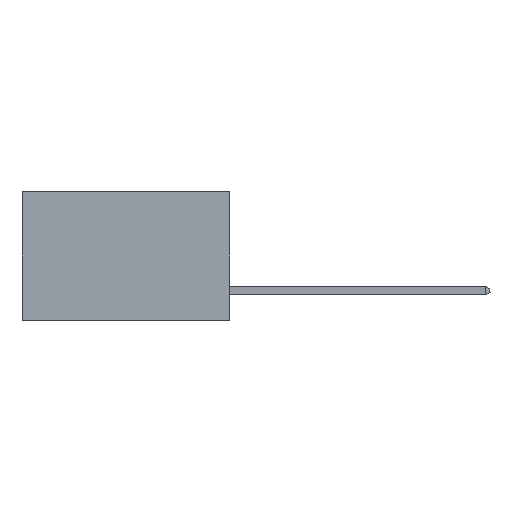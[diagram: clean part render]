
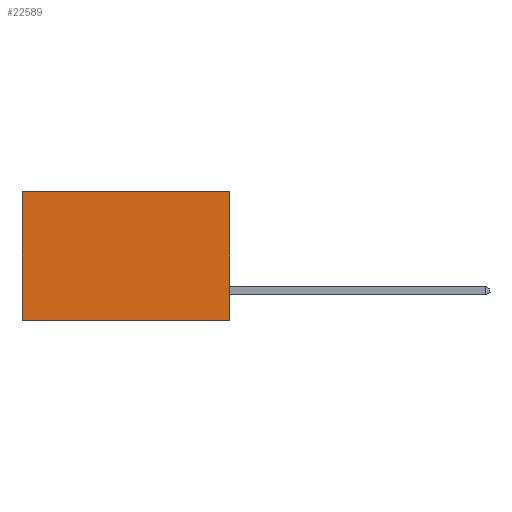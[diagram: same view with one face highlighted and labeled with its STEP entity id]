
A CAD part, left-side view. The second image highlights one B-rep face of the part: STEP entity #22589.
In plain terms, the highlighted planar face has unit normal (-1, 0, 0).
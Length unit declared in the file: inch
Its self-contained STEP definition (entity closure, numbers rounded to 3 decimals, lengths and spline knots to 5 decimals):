
#183 = CARTESIAN_POINT ( 'NONE',  ( 0.298, 0., 0. ) ) ;
#554 = ORIENTED_EDGE ( 'NONE', *, *, #14178, .T. ) ;
#616 = VECTOR ( 'NONE', #5050, 39.37008 ) ;
#893 = LINE ( 'NONE', #14242, #616 ) ;
#899 = DIRECTION ( 'NONE',  ( 0., 1., 0. ) ) ;
#2391 = EDGE_LOOP ( 'NONE', ( #554, #18016, #14840, #8292 ) ) ;
#2414 = VECTOR ( 'NONE', #12637, 39.37008 ) ;
#2501 = VECTOR ( 'NONE', #899, 39.37008 ) ;
#2810 = EDGE_CURVE ( 'NONE', #11229, #7564, #893, .T. ) ;
#3597 = CARTESIAN_POINT ( 'NONE',  ( 0.298, 0.6, -0.37 ) ) ;
#3618 = LINE ( 'NONE', #6335, #2501 ) ;
#3905 = DIRECTION ( 'NONE',  ( 0., 0., -1. ) ) ;
#5050 = DIRECTION ( 'NONE',  ( 0., 0., -1. ) ) ;
#5509 = CARTESIAN_POINT ( 'NONE',  ( 0.298, 0., -0.37 ) ) ;
#6335 = CARTESIAN_POINT ( 'NONE',  ( 0.298, 0., -0.37 ) ) ;
#6349 = VERTEX_POINT ( 'NONE', #15378 ) ;
#7564 = VERTEX_POINT ( 'NONE', #5509 ) ;
#8292 = ORIENTED_EDGE ( 'NONE', *, *, #21353, .T. ) ;
#8695 = CARTESIAN_POINT ( 'NONE',  ( 0.298, 0.6, 0. ) ) ;
#9475 = EDGE_CURVE ( 'NONE', #7564, #16590, #3618, .T. ) ;
#10483 = LINE ( 'NONE', #183, #2414 ) ;
#11229 = VERTEX_POINT ( 'NONE', #15249 ) ;
#11423 = LINE ( 'NONE', #8695, #19980 ) ;
#12637 = DIRECTION ( 'NONE',  ( 0., 1., 0. ) ) ;
#14178 = EDGE_CURVE ( 'NONE', #6349, #16590, #11423, .T. ) ;
#14242 = CARTESIAN_POINT ( 'NONE',  ( 0.298, 0., 0. ) ) ;
#14420 = DIRECTION ( 'NONE',  ( 1., 0., 0. ) ) ;
#14840 = ORIENTED_EDGE ( 'NONE', *, *, #2810, .F. ) ;
#15249 = CARTESIAN_POINT ( 'NONE',  ( 0.298, 0., 0. ) ) ;
#15378 = CARTESIAN_POINT ( 'NONE',  ( 0.298, 0.6, 0. ) ) ;
#16590 = VERTEX_POINT ( 'NONE', #3597 ) ;
#18016 = ORIENTED_EDGE ( 'NONE', *, *, #9475, .F. ) ;
#19766 = PLANE ( 'NONE',  #21239 ) ;
#19980 = VECTOR ( 'NONE', #21079, 39.37008 ) ;
#20131 = FACE_OUTER_BOUND ( 'NONE', #2391, .T. ) ;
#21079 = DIRECTION ( 'NONE',  ( 0., 0., -1. ) ) ;
#21239 = AXIS2_PLACEMENT_3D ( 'NONE', #21653, #14420, #3905 ) ;
#21353 = EDGE_CURVE ( 'NONE', #11229, #6349, #10483, .T. ) ;
#21653 = CARTESIAN_POINT ( 'NONE',  ( 0.298, 0., 0. ) ) ;
#22589 = ADVANCED_FACE ( 'NONE', ( #20131 ), #19766, .F. ) ;
